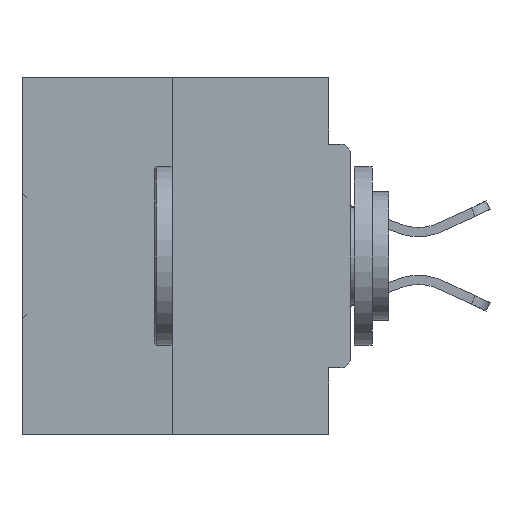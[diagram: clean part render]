
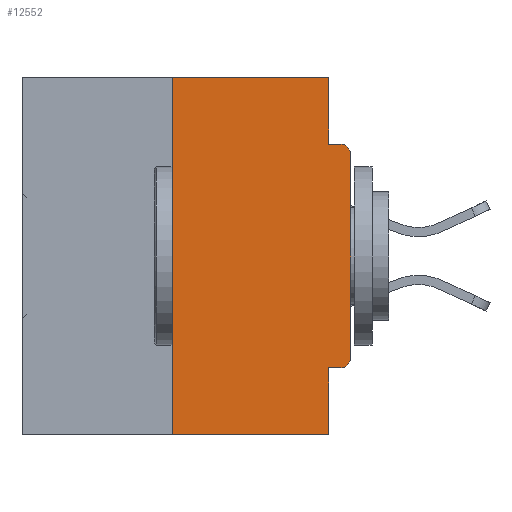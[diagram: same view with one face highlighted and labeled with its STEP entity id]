
A CAD part, left-side view. The second image highlights one B-rep face of the part: STEP entity #12552.
In plain terms, the highlighted planar face has unit normal (-1, 0, 0).
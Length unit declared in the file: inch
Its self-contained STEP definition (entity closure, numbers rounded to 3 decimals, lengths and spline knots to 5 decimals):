
#109 = CARTESIAN_POINT ( 'NONE',  ( 0., 0., -0.4065 ) ) ;
#535 = AXIS2_PLACEMENT_3D ( 'NONE', #4599, #33127, #8200 ) ;
#676 = DIRECTION ( 'NONE',  ( 0., -1., 0. ) ) ;
#2460 = EDGE_CURVE ( 'NONE', #21637, #19778, #24589, .T. ) ;
#3041 = EDGE_CURVE ( 'NONE', #21153, #19873, #12113, .T. ) ;
#3349 = DIRECTION ( 'NONE',  ( 0., -1., 0. ) ) ;
#4279 = EDGE_CURVE ( 'NONE', #5868, #19778, #36850, .T. ) ;
#4599 = CARTESIAN_POINT ( 'NONE',  ( 0., 0.015, -0.1085 ) ) ;
#4613 = LINE ( 'NONE', #41948, #32246 ) ;
#5071 = AXIS2_PLACEMENT_3D ( 'NONE', #14702, #26019, #18471 ) ;
#5868 = VERTEX_POINT ( 'NONE', #16210 ) ;
#6211 = LINE ( 'NONE', #109, #42369 ) ;
#6575 = DIRECTION ( 'NONE',  ( 0., 0., 1. ) ) ;
#6799 = CARTESIAN_POINT ( 'NONE',  ( 0., 0.46, 0. ) ) ;
#6835 = DIRECTION ( 'NONE',  ( 0., 0., -1. ) ) ;
#7744 = ORIENTED_EDGE ( 'NONE', *, *, #25269, .T. ) ;
#7847 = ORIENTED_EDGE ( 'NONE', *, *, #11830, .F. ) ;
#8200 = DIRECTION ( 'NONE',  ( 0., 0., -1. ) ) ;
#9658 = CARTESIAN_POINT ( 'NONE',  ( 0., 0.031, -0.5 ) ) ;
#10414 = DIRECTION ( 'NONE',  ( 0., -1., 0. ) ) ;
#10456 = EDGE_CURVE ( 'NONE', #21153, #44090, #6211, .T. ) ;
#10803 = DIRECTION ( 'NONE',  ( 0., 1., 0. ) ) ;
#11450 = VERTEX_POINT ( 'NONE', #19037 ) ;
#11725 = EDGE_CURVE ( 'NONE', #26788, #11450, #46583, .T. ) ;
#11830 = EDGE_CURVE ( 'NONE', #44090, #44378, #14920, .T. ) ;
#12113 = CIRCLE ( 'NONE', #37752, 0.015 ) ;
#12552 = ADVANCED_FACE ( 'NONE', ( #39116 ), #29178, .F. ) ;
#14234 = CARTESIAN_POINT ( 'NONE',  ( 0., 0.46, -0.5 ) ) ;
#14702 = CARTESIAN_POINT ( 'NONE',  ( 0., 0.46, 0. ) ) ;
#14920 = LINE ( 'NONE', #43304, #17180 ) ;
#15511 = VECTOR ( 'NONE', #46012, 39.37008 ) ;
#15995 = ORIENTED_EDGE ( 'NONE', *, *, #19020, .T. ) ;
#16210 = CARTESIAN_POINT ( 'NONE',  ( 0., 0.031, -0.0935 ) ) ;
#17180 = VECTOR ( 'NONE', #6835, 39.37008 ) ;
#18471 = DIRECTION ( 'NONE',  ( 0., 0., -1. ) ) ;
#19014 = EDGE_CURVE ( 'NONE', #11450, #25565, #20428, .T. ) ;
#19020 = EDGE_CURVE ( 'NONE', #26788, #44378, #32792, .T. ) ;
#19037 = CARTESIAN_POINT ( 'NONE',  ( 0., 0.25, 0. ) ) ;
#19778 = VERTEX_POINT ( 'NONE', #44792 ) ;
#19820 = ORIENTED_EDGE ( 'NONE', *, *, #44679, .F. ) ;
#19873 = VERTEX_POINT ( 'NONE', #44483 ) ;
#20428 = LINE ( 'NONE', #6799, #29413 ) ;
#20934 = CARTESIAN_POINT ( 'NONE',  ( 0., 0.25, -0.5 ) ) ;
#21016 = ORIENTED_EDGE ( 'NONE', *, *, #4279, .F. ) ;
#21153 = VERTEX_POINT ( 'NONE', #21387 ) ;
#21387 = CARTESIAN_POINT ( 'NONE',  ( 0., 0.015, -0.4065 ) ) ;
#21637 = VERTEX_POINT ( 'NONE', #27168 ) ;
#24589 = CIRCLE ( 'NONE', #535, 0.015 ) ;
#25269 = EDGE_CURVE ( 'NONE', #19873, #21637, #45170, .T. ) ;
#25525 = EDGE_LOOP ( 'NONE', ( #37622, #45092, #15995, #7847, #36877, #29585, #7744, #44133, #21016, #19820 ) ) ;
#25565 = VERTEX_POINT ( 'NONE', #40507 ) ;
#26019 = DIRECTION ( 'NONE',  ( 1., 0., 0. ) ) ;
#26240 = CARTESIAN_POINT ( 'NONE',  ( 0., 0.031, -0.4065 ) ) ;
#26788 = VERTEX_POINT ( 'NONE', #20934 ) ;
#27168 = CARTESIAN_POINT ( 'NONE',  ( 0., 0., -0.1085 ) ) ;
#27537 = CARTESIAN_POINT ( 'NONE',  ( 0., 0.015, -0.3915 ) ) ;
#29178 = PLANE ( 'NONE',  #5071 ) ;
#29413 = VECTOR ( 'NONE', #10414, 39.37008 ) ;
#29585 = ORIENTED_EDGE ( 'NONE', *, *, #3041, .T. ) ;
#32246 = VECTOR ( 'NONE', #42268, 39.37008 ) ;
#32708 = VECTOR ( 'NONE', #6575, 39.37008 ) ;
#32792 = LINE ( 'NONE', #14234, #38472 ) ;
#33127 = DIRECTION ( 'NONE',  ( -1., 0., 0. ) ) ;
#35279 = CARTESIAN_POINT ( 'NONE',  ( 0., 0., 0. ) ) ;
#36850 = LINE ( 'NONE', #40260, #39134 ) ;
#36877 = ORIENTED_EDGE ( 'NONE', *, *, #10456, .F. ) ;
#37622 = ORIENTED_EDGE ( 'NONE', *, *, #19014, .F. ) ;
#37752 = AXIS2_PLACEMENT_3D ( 'NONE', #27537, #38116, #41614 ) ;
#38116 = DIRECTION ( 'NONE',  ( -1., 0., 0. ) ) ;
#38472 = VECTOR ( 'NONE', #3349, 39.37008 ) ;
#39116 = FACE_OUTER_BOUND ( 'NONE', #25525, .T. ) ;
#39134 = VECTOR ( 'NONE', #676, 39.37008 ) ;
#40260 = CARTESIAN_POINT ( 'NONE',  ( 0., 0., -0.0935 ) ) ;
#40507 = CARTESIAN_POINT ( 'NONE',  ( 0., 0.031, 0. ) ) ;
#41614 = DIRECTION ( 'NONE',  ( 0., 0., -1. ) ) ;
#41948 = CARTESIAN_POINT ( 'NONE',  ( 0., 0.031, 0. ) ) ;
#42268 = DIRECTION ( 'NONE',  ( 0., 0., -1. ) ) ;
#42369 = VECTOR ( 'NONE', #10803, 39.37008 ) ;
#43304 = CARTESIAN_POINT ( 'NONE',  ( 0., 0.031, -0.5 ) ) ;
#44090 = VERTEX_POINT ( 'NONE', #26240 ) ;
#44133 = ORIENTED_EDGE ( 'NONE', *, *, #2460, .T. ) ;
#44378 = VERTEX_POINT ( 'NONE', #9658 ) ;
#44483 = CARTESIAN_POINT ( 'NONE',  ( 0., 0., -0.3915 ) ) ;
#44679 = EDGE_CURVE ( 'NONE', #25565, #5868, #4613, .T. ) ;
#44792 = CARTESIAN_POINT ( 'NONE',  ( 0., 0.015, -0.0935 ) ) ;
#45092 = ORIENTED_EDGE ( 'NONE', *, *, #11725, .F. ) ;
#45170 = LINE ( 'NONE', #35279, #32708 ) ;
#45854 = CARTESIAN_POINT ( 'NONE',  ( 0., 0.25, 0. ) ) ;
#46012 = DIRECTION ( 'NONE',  ( 0., 0., 1. ) ) ;
#46583 = LINE ( 'NONE', #45854, #15511 ) ;
